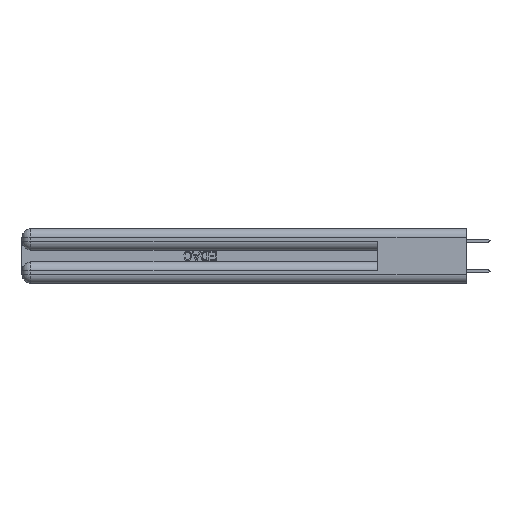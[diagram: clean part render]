
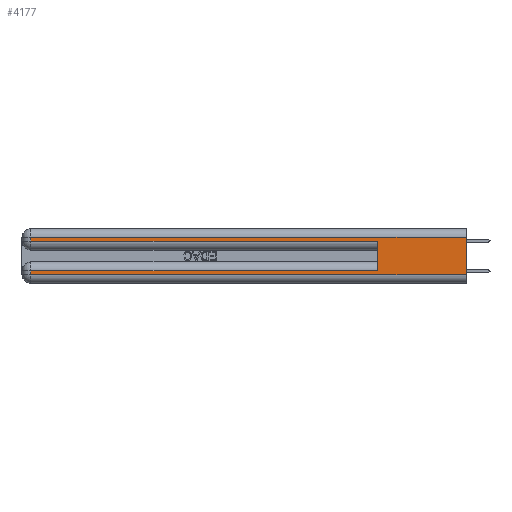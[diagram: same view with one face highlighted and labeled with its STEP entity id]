
A CAD part, left-side view. The second image highlights one B-rep face of the part: STEP entity #4177.
In plain terms, the highlighted planar face has unit normal (-1, 0, 0).
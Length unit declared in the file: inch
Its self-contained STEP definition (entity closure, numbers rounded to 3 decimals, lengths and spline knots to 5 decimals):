
#1108 = VERTEX_POINT ( 'NONE', #35987 ) ;
#1827 = VECTOR ( 'NONE', #5325, 39.37008 ) ;
#2268 = DIRECTION ( 'NONE',  ( 0., 0., -1. ) ) ;
#2497 = EDGE_CURVE ( 'NONE', #21753, #43687, #49968, .T. ) ;
#3309 = ORIENTED_EDGE ( 'NONE', *, *, #5769, .F. ) ;
#3467 = EDGE_CURVE ( 'NONE', #43687, #30939, #35266, .T. ) ;
#4177 = ADVANCED_FACE ( 'NONE', ( #25004 ), #21761, .F. ) ;
#4189 = DIRECTION ( 'NONE',  ( 0., -1., 0. ) ) ;
#4462 = DIRECTION ( 'NONE',  ( 0., 0., -1. ) ) ;
#4667 = LINE ( 'NONE', #13149, #24232 ) ;
#5325 = DIRECTION ( 'NONE',  ( 0., 1., 0. ) ) ;
#5769 = EDGE_CURVE ( 'NONE', #14361, #39346, #4667, .T. ) ;
#6854 = VERTEX_POINT ( 'NONE', #42903 ) ;
#8095 = VECTOR ( 'NONE', #2268, 39.37008 ) ;
#9054 = ORIENTED_EDGE ( 'NONE', *, *, #28095, .T. ) ;
#9681 = ORIENTED_EDGE ( 'NONE', *, *, #31495, .T. ) ;
#10088 = DIRECTION ( 'NONE',  ( 0., 0., -1. ) ) ;
#10144 = CARTESIAN_POINT ( 'NONE',  ( 0., 0., 0.285 ) ) ;
#10221 = EDGE_CURVE ( 'NONE', #6854, #39346, #17471, .T. ) ;
#11694 = VECTOR ( 'NONE', #22456, 39.37008 ) ;
#12205 = LINE ( 'NONE', #20729, #1827 ) ;
#13149 = CARTESIAN_POINT ( 'NONE',  ( 0., 0., 0.37 ) ) ;
#14096 = DIRECTION ( 'NONE',  ( 0., -1., 0. ) ) ;
#14361 = VERTEX_POINT ( 'NONE', #27547 ) ;
#14438 = CARTESIAN_POINT ( 'NONE',  ( 0., 2.94, 0.31 ) ) ;
#15505 = LINE ( 'NONE', #46568, #24666 ) ;
#15820 = CARTESIAN_POINT ( 'NONE',  ( 0., 0., 0.06 ) ) ;
#17089 = DIRECTION ( 'NONE',  ( 0., 0., -1. ) ) ;
#17471 = LINE ( 'NONE', #15820, #27806 ) ;
#17608 = VECTOR ( 'NONE', #4462, 39.37008 ) ;
#18542 = CARTESIAN_POINT ( 'NONE',  ( 0., 0.6, 0.145 ) ) ;
#20729 = CARTESIAN_POINT ( 'NONE',  ( 0., 0., 0.31 ) ) ;
#21753 = VERTEX_POINT ( 'NONE', #14438 ) ;
#21761 = PLANE ( 'NONE',  #48497 ) ;
#22129 = LINE ( 'NONE', #18542, #11694 ) ;
#22456 = DIRECTION ( 'NONE',  ( 0., 0., 1. ) ) ;
#22542 = ORIENTED_EDGE ( 'NONE', *, *, #10221, .T. ) ;
#24232 = VECTOR ( 'NONE', #17089, 39.37008 ) ;
#24666 = VECTOR ( 'NONE', #27074, 39.37008 ) ;
#24887 = VECTOR ( 'NONE', #14096, 39.37008 ) ;
#25004 = FACE_OUTER_BOUND ( 'NONE', #46115, .T. ) ;
#27074 = DIRECTION ( 'NONE',  ( 0., 1., 0. ) ) ;
#27547 = CARTESIAN_POINT ( 'NONE',  ( 0., 0., 0.31 ) ) ;
#27806 = VECTOR ( 'NONE', #4189, 39.37008 ) ;
#27838 = CARTESIAN_POINT ( 'NONE',  ( 0., 2.94, 0.37 ) ) ;
#28095 = EDGE_CURVE ( 'NONE', #14361, #21753, #12205, .T. ) ;
#29109 = CARTESIAN_POINT ( 'NONE',  ( 0., 2.94, 0.285 ) ) ;
#29229 = ORIENTED_EDGE ( 'NONE', *, *, #2497, .T. ) ;
#29560 = CARTESIAN_POINT ( 'NONE',  ( 0., 0., 0.37 ) ) ;
#29579 = CARTESIAN_POINT ( 'NONE',  ( 0., 2.94, 0.37 ) ) ;
#30939 = VERTEX_POINT ( 'NONE', #33728 ) ;
#31495 = EDGE_CURVE ( 'NONE', #1108, #6854, #39242, .T. ) ;
#31881 = EDGE_CURVE ( 'NONE', #33480, #30939, #22129, .T. ) ;
#33480 = VERTEX_POINT ( 'NONE', #47236 ) ;
#33481 = DIRECTION ( 'NONE',  ( 1., 0., 0. ) ) ;
#33728 = CARTESIAN_POINT ( 'NONE',  ( 0., 0.6, 0.285 ) ) ;
#35266 = LINE ( 'NONE', #10144, #24887 ) ;
#35987 = CARTESIAN_POINT ( 'NONE',  ( 0., 2.94, 0.085 ) ) ;
#37167 = ORIENTED_EDGE ( 'NONE', *, *, #3467, .T. ) ;
#39242 = LINE ( 'NONE', #29579, #8095 ) ;
#39346 = VERTEX_POINT ( 'NONE', #50335 ) ;
#42903 = CARTESIAN_POINT ( 'NONE',  ( 0., 2.94, 0.06 ) ) ;
#43337 = EDGE_CURVE ( 'NONE', #33480, #1108, #15505, .T. ) ;
#43687 = VERTEX_POINT ( 'NONE', #29109 ) ;
#43884 = ORIENTED_EDGE ( 'NONE', *, *, #43337, .T. ) ;
#46115 = EDGE_LOOP ( 'NONE', ( #3309, #9054, #29229, #37167, #46345, #43884, #9681, #22542 ) ) ;
#46345 = ORIENTED_EDGE ( 'NONE', *, *, #31881, .F. ) ;
#46568 = CARTESIAN_POINT ( 'NONE',  ( 0., 0., 0.085 ) ) ;
#47236 = CARTESIAN_POINT ( 'NONE',  ( 0., 0.6, 0.085 ) ) ;
#48497 = AXIS2_PLACEMENT_3D ( 'NONE', #29560, #33481, #10088 ) ;
#49968 = LINE ( 'NONE', #27838, #17608 ) ;
#50335 = CARTESIAN_POINT ( 'NONE',  ( 0., 0., 0.06 ) ) ;
